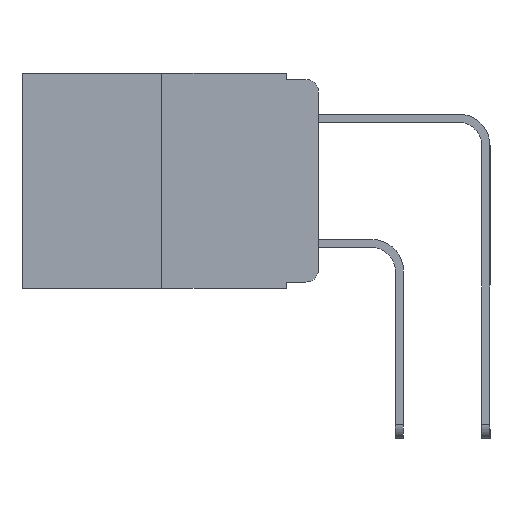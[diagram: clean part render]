
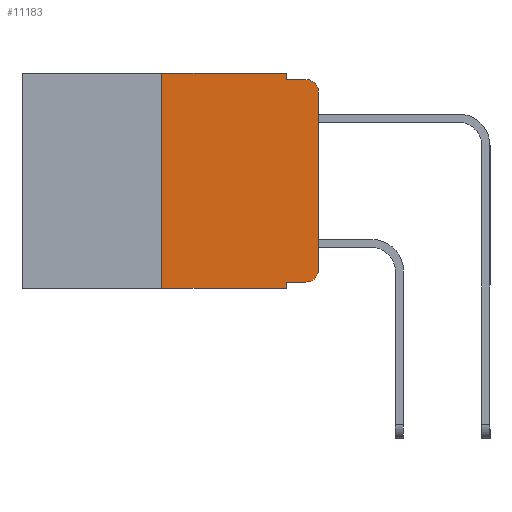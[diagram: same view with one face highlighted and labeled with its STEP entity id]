
A CAD part, left-side view. The second image highlights one B-rep face of the part: STEP entity #11183.
In plain terms, the highlighted planar face has unit normal (-1, 0, 0).
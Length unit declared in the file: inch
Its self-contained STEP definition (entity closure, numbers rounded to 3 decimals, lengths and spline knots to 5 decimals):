
#92 = VECTOR ( 'NONE', #20238, 39.37008 ) ;
#173 = VECTOR ( 'NONE', #24779, 39.37008 ) ;
#326 = DIRECTION ( 'NONE',  ( 0., 0., -1. ) ) ;
#399 = EDGE_CURVE ( 'NONE', #7493, #12326, #21824, .T. ) ;
#730 = VERTEX_POINT ( 'NONE', #23235 ) ;
#761 = LINE ( 'NONE', #17676, #20738 ) ;
#1013 = CIRCLE ( 'NONE', #4351, 0.02 ) ;
#1327 = VECTOR ( 'NONE', #14632, 39.37008 ) ;
#2153 = ORIENTED_EDGE ( 'NONE', *, *, #16675, .F. ) ;
#2581 = CARTESIAN_POINT ( 'NONE',  ( 0., 0.051, -0.333 ) ) ;
#2899 = CARTESIAN_POINT ( 'NONE',  ( 0., 0.051, -0.01 ) ) ;
#3295 = CARTESIAN_POINT ( 'NONE',  ( 0., 0.25, -0.343 ) ) ;
#3417 = ORIENTED_EDGE ( 'NONE', *, *, #5643, .F. ) ;
#4351 = AXIS2_PLACEMENT_3D ( 'NONE', #18230, #6791, #20122 ) ;
#4367 = CARTESIAN_POINT ( 'NONE',  ( 0., 0.051, 0. ) ) ;
#4985 = PLANE ( 'NONE',  #23457 ) ;
#5401 = DIRECTION ( 'NONE',  ( 0., 0., 1. ) ) ;
#5643 = EDGE_CURVE ( 'NONE', #7493, #17378, #20155, .T. ) ;
#5740 = CARTESIAN_POINT ( 'NONE',  ( 0., 0.02, -0.313 ) ) ;
#6444 = DIRECTION ( 'NONE',  ( 0., 0., -1. ) ) ;
#6727 = EDGE_CURVE ( 'NONE', #22683, #8089, #11216, .T. ) ;
#6791 = DIRECTION ( 'NONE',  ( -1., 0., 0. ) ) ;
#6826 = VERTEX_POINT ( 'NONE', #12902 ) ;
#6955 = DIRECTION ( 'NONE',  ( 0., 0., -1. ) ) ;
#7433 = ORIENTED_EDGE ( 'NONE', *, *, #20787, .F. ) ;
#7473 = CARTESIAN_POINT ( 'NONE',  ( 0., 0.051, 0. ) ) ;
#7493 = VERTEX_POINT ( 'NONE', #3295 ) ;
#7695 = DIRECTION ( 'NONE',  ( 0., 0., -1. ) ) ;
#7807 = EDGE_CURVE ( 'NONE', #6826, #15099, #18313, .T. ) ;
#8089 = VERTEX_POINT ( 'NONE', #9359 ) ;
#8635 = ORIENTED_EDGE ( 'NONE', *, *, #399, .T. ) ;
#9249 = ORIENTED_EDGE ( 'NONE', *, *, #24203, .F. ) ;
#9359 = CARTESIAN_POINT ( 'NONE',  ( 0., 0.02, -0.01 ) ) ;
#9529 = ORIENTED_EDGE ( 'NONE', *, *, #10073, .T. ) ;
#9826 = ORIENTED_EDGE ( 'NONE', *, *, #7807, .T. ) ;
#10024 = VECTOR ( 'NONE', #5401, 39.37008 ) ;
#10073 = EDGE_CURVE ( 'NONE', #19020, #8089, #1013, .T. ) ;
#10692 = LINE ( 'NONE', #22883, #173 ) ;
#10929 = CIRCLE ( 'NONE', #12975, 0.02 ) ;
#11103 = CARTESIAN_POINT ( 'NONE',  ( 0., 0., -0.03 ) ) ;
#11112 = LINE ( 'NONE', #24238, #11710 ) ;
#11183 = ADVANCED_FACE ( 'NONE', ( #11694 ), #4985, .F. ) ;
#11216 = LINE ( 'NONE', #2899, #92 ) ;
#11694 = FACE_OUTER_BOUND ( 'NONE', #24332, .T. ) ;
#11710 = VECTOR ( 'NONE', #12848, 39.37008 ) ;
#12265 = DIRECTION ( 'NONE',  ( 0., -1., 0. ) ) ;
#12326 = VERTEX_POINT ( 'NONE', #14340 ) ;
#12338 = LINE ( 'NONE', #4367, #16815 ) ;
#12848 = DIRECTION ( 'NONE',  ( 0., -1., 0. ) ) ;
#12902 = CARTESIAN_POINT ( 'NONE',  ( 0., 0.051, -0.333 ) ) ;
#12975 = AXIS2_PLACEMENT_3D ( 'NONE', #5740, #19127, #7695 ) ;
#14340 = CARTESIAN_POINT ( 'NONE',  ( 0., 0.051, -0.343 ) ) ;
#14632 = DIRECTION ( 'NONE',  ( 0., -1., 0. ) ) ;
#14904 = ORIENTED_EDGE ( 'NONE', *, *, #22481, .T. ) ;
#15099 = VERTEX_POINT ( 'NONE', #22302 ) ;
#15855 = CARTESIAN_POINT ( 'NONE',  ( 0., 0.051, -0.01 ) ) ;
#16536 = CARTESIAN_POINT ( 'NONE',  ( 0., 0.473, -0.343 ) ) ;
#16675 = EDGE_CURVE ( 'NONE', #19671, #22683, #761, .T. ) ;
#16815 = VECTOR ( 'NONE', #6444, 39.37008 ) ;
#17378 = VERTEX_POINT ( 'NONE', #22877 ) ;
#17676 = CARTESIAN_POINT ( 'NONE',  ( 0., 0.051, 0. ) ) ;
#18230 = CARTESIAN_POINT ( 'NONE',  ( 0., 0.02, -0.03 ) ) ;
#18313 = LINE ( 'NONE', #2581, #23341 ) ;
#18407 = DIRECTION ( 'NONE',  ( 1., 0., 0. ) ) ;
#19020 = VERTEX_POINT ( 'NONE', #11103 ) ;
#19127 = DIRECTION ( 'NONE',  ( -1., 0., 0. ) ) ;
#19650 = ORIENTED_EDGE ( 'NONE', *, *, #6727, .F. ) ;
#19671 = VERTEX_POINT ( 'NONE', #7473 ) ;
#20122 = DIRECTION ( 'NONE',  ( 0., 0., -1. ) ) ;
#20155 = LINE ( 'NONE', #24502, #10024 ) ;
#20238 = DIRECTION ( 'NONE',  ( 0., -1., 0. ) ) ;
#20738 = VECTOR ( 'NONE', #326, 39.37008 ) ;
#20787 = EDGE_CURVE ( 'NONE', #17378, #19671, #11112, .T. ) ;
#21348 = EDGE_CURVE ( 'NONE', #730, #19020, #10692, .T. ) ;
#21824 = LINE ( 'NONE', #16536, #1327 ) ;
#22302 = CARTESIAN_POINT ( 'NONE',  ( 0., 0.02, -0.333 ) ) ;
#22481 = EDGE_CURVE ( 'NONE', #15099, #730, #10929, .T. ) ;
#22683 = VERTEX_POINT ( 'NONE', #15855 ) ;
#22877 = CARTESIAN_POINT ( 'NONE',  ( 0., 0.25, 0. ) ) ;
#22883 = CARTESIAN_POINT ( 'NONE',  ( 0., 0., 0. ) ) ;
#22908 = ORIENTED_EDGE ( 'NONE', *, *, #21348, .T. ) ;
#23235 = CARTESIAN_POINT ( 'NONE',  ( 0., 0., -0.313 ) ) ;
#23341 = VECTOR ( 'NONE', #12265, 39.37008 ) ;
#23457 = AXIS2_PLACEMENT_3D ( 'NONE', #24040, #18407, #6955 ) ;
#24040 = CARTESIAN_POINT ( 'NONE',  ( 0., 0.473, 0. ) ) ;
#24203 = EDGE_CURVE ( 'NONE', #6826, #12326, #12338, .T. ) ;
#24238 = CARTESIAN_POINT ( 'NONE',  ( 0., 0.473, 0. ) ) ;
#24332 = EDGE_LOOP ( 'NONE', ( #22908, #9529, #19650, #2153, #7433, #3417, #8635, #9249, #9826, #14904 ) ) ;
#24502 = CARTESIAN_POINT ( 'NONE',  ( 0., 0.25, 0. ) ) ;
#24779 = DIRECTION ( 'NONE',  ( 0., 0., 1. ) ) ;
